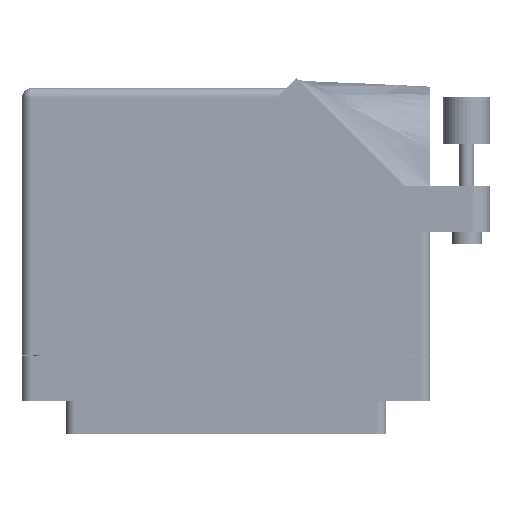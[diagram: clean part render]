
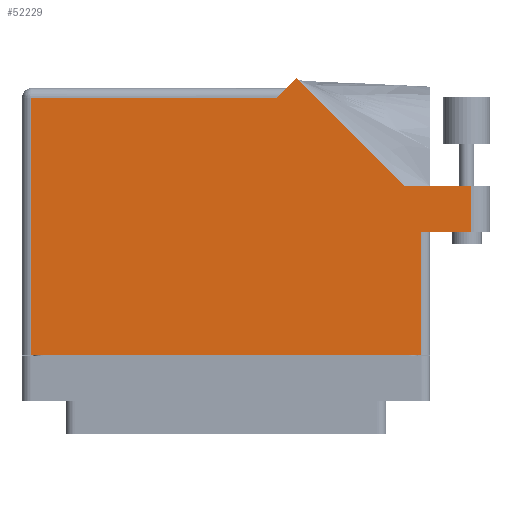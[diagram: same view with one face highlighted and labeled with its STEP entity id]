
A CAD part, front view. The second image highlights one B-rep face of the part: STEP entity #52229.
In plain terms, the highlighted face is planar.
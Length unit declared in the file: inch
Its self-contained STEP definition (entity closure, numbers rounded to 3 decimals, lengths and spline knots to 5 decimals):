
#177 = CARTESIAN_POINT ( 'NONE',  ( 0.46971, 1.74571, 0.617 ) ) ;
#880 = CARTESIAN_POINT ( 'NONE',  ( -1.359, -0.1, 0.617 ) ) ;
#1022 = EDGE_CURVE ( 'NONE', #62810, #7657, #22657, .T. ) ;
#1053 = CARTESIAN_POINT ( 'NONE',  ( -1.297, 1.613, 0.617 ) ) ;
#2074 = CARTESIAN_POINT ( 'NONE',  ( 0.337, 1.613, 0.617 ) ) ;
#2374 = ORIENTED_EDGE ( 'NONE', *, *, #52291, .T. ) ;
#2992 = ORIENTED_EDGE ( 'NONE', *, *, #36825, .T. ) ;
#3361 = LINE ( 'NONE', #880, #59440 ) ;
#3631 = CARTESIAN_POINT ( 'NONE',  ( 1.19342, 1.022, 0.617 ) ) ;
#3835 = LINE ( 'NONE', #46637, #49665 ) ;
#4094 = VERTEX_POINT ( 'NONE', #69458 ) ;
#4654 = EDGE_CURVE ( 'NONE', #60311, #33044, #35469, .T. ) ;
#4778 = ORIENTED_EDGE ( 'NONE', *, *, #31855, .T. ) ;
#5487 = VECTOR ( 'NONE', #17657, 39.37008 ) ;
#6128 = LINE ( 'NONE', #58465, #59645 ) ;
#6171 = CARTESIAN_POINT ( 'NONE',  ( -1.359, 1.675, 0.617 ) ) ;
#6475 = ORIENTED_EDGE ( 'NONE', *, *, #55195, .T. ) ;
#7368 = EDGE_CURVE ( 'NONE', #4094, #60311, #11407, .T. ) ;
#7657 = VERTEX_POINT ( 'NONE', #1053 ) ;
#7923 = AXIS2_PLACEMENT_3D ( 'NONE', #6171, #37727, #27763 ) ;
#8022 = DIRECTION ( 'NONE',  ( -0.707, -0.707, 0. ) ) ;
#10796 = CARTESIAN_POINT ( 'NONE',  ( 1.297, 0.715, 0.617 ) ) ;
#11407 = LINE ( 'NONE', #41815, #5487 ) ;
#14910 = LINE ( 'NONE', #33439, #36952 ) ;
#15592 = ORIENTED_EDGE ( 'NONE', *, *, #4654, .T. ) ;
#17074 = PLANE ( 'NONE',  #7923 ) ;
#17657 = DIRECTION ( 'NONE',  ( -1., 0., 0. ) ) ;
#18263 = CARTESIAN_POINT ( 'NONE',  ( 1.19342, 1.022, 0.617 ) ) ;
#18620 = VECTOR ( 'NONE', #52535, 39.37008 ) ;
#22469 = CARTESIAN_POINT ( 'NONE',  ( 1.359, 0.715, 0.617 ) ) ;
#22657 = LINE ( 'NONE', #40861, #48982 ) ;
#25996 = VERTEX_POINT ( 'NONE', #70314 ) ;
#27763 = DIRECTION ( 'NONE',  ( -1., 0., 0. ) ) ;
#28224 = VECTOR ( 'NONE', #50427, 39.37008 ) ;
#29945 = CARTESIAN_POINT ( 'NONE',  ( 1.297, -0.1, 0.617 ) ) ;
#30753 = VECTOR ( 'NONE', #45112, 39.37008 ) ;
#31855 = EDGE_CURVE ( 'NONE', #43001, #4094, #6128, .T. ) ;
#33044 = VERTEX_POINT ( 'NONE', #177 ) ;
#33072 = ORIENTED_EDGE ( 'NONE', *, *, #66696, .T. ) ;
#33439 = CARTESIAN_POINT ( 'NONE',  ( -1.297, -0.1, 0.617 ) ) ;
#34406 = DIRECTION ( 'NONE',  ( 0., -1., 0. ) ) ;
#35387 = VERTEX_POINT ( 'NONE', #63617 ) ;
#35469 = LINE ( 'NONE', #3631, #18620 ) ;
#36139 = FACE_OUTER_BOUND ( 'NONE', #67970, .T. ) ;
#36825 = EDGE_CURVE ( 'NONE', #25996, #43001, #40130, .T. ) ;
#36952 = VECTOR ( 'NONE', #34406, 39.37008 ) ;
#37727 = DIRECTION ( 'NONE',  ( 0., 0., -1. ) ) ;
#40130 = LINE ( 'NONE', #22469, #28224 ) ;
#40861 = CARTESIAN_POINT ( 'NONE',  ( -1.359, 1.613, 0.617 ) ) ;
#41815 = CARTESIAN_POINT ( 'NONE',  ( 1.759, 1.022, 0.617 ) ) ;
#43001 = VERTEX_POINT ( 'NONE', #66863 ) ;
#45112 = DIRECTION ( 'NONE',  ( 0., 1., 0. ) ) ;
#46322 = ORIENTED_EDGE ( 'NONE', *, *, #1022, .T. ) ;
#46637 = CARTESIAN_POINT ( 'NONE',  ( 0.399, 1.675, 0.617 ) ) ;
#47023 = DIRECTION ( 'NONE',  ( 0., 1., 0. ) ) ;
#48982 = VECTOR ( 'NONE', #62781, 39.37008 ) ;
#49665 = VECTOR ( 'NONE', #8022, 39.37008 ) ;
#50427 = DIRECTION ( 'NONE',  ( 1., 0., 0. ) ) ;
#52229 = ADVANCED_FACE ( 'NONE', ( #36139 ), #17074, .F. ) ;
#52291 = EDGE_CURVE ( 'NONE', #7657, #35387, #14910, .T. ) ;
#52535 = DIRECTION ( 'NONE',  ( -0.707, 0.707, 0. ) ) ;
#55195 = EDGE_CURVE ( 'NONE', #58256, #25996, #59667, .T. ) ;
#55841 = ORIENTED_EDGE ( 'NONE', *, *, #7368, .T. ) ;
#55918 = EDGE_CURVE ( 'NONE', #33044, #62810, #3835, .T. ) ;
#57486 = DIRECTION ( 'NONE',  ( 1., 0., 0. ) ) ;
#58256 = VERTEX_POINT ( 'NONE', #29945 ) ;
#58465 = CARTESIAN_POINT ( 'NONE',  ( 1.634, 1.022, 0.617 ) ) ;
#59440 = VECTOR ( 'NONE', #57486, 39.37008 ) ;
#59645 = VECTOR ( 'NONE', #47023, 39.37008 ) ;
#59667 = LINE ( 'NONE', #10796, #30753 ) ;
#60311 = VERTEX_POINT ( 'NONE', #18263 ) ;
#62781 = DIRECTION ( 'NONE',  ( -1., 0., 0. ) ) ;
#62810 = VERTEX_POINT ( 'NONE', #2074 ) ;
#63617 = CARTESIAN_POINT ( 'NONE',  ( -1.297, -0.1, 0.617 ) ) ;
#66696 = EDGE_CURVE ( 'NONE', #35387, #58256, #3361, .T. ) ;
#66863 = CARTESIAN_POINT ( 'NONE',  ( 1.634, 0.715, 0.617 ) ) ;
#67970 = EDGE_LOOP ( 'NONE', ( #2992, #4778, #55841, #15592, #70456, #46322, #2374, #33072, #6475 ) ) ;
#69458 = CARTESIAN_POINT ( 'NONE',  ( 1.634, 1.022, 0.617 ) ) ;
#70314 = CARTESIAN_POINT ( 'NONE',  ( 1.297, 0.715, 0.617 ) ) ;
#70456 = ORIENTED_EDGE ( 'NONE', *, *, #55918, .T. ) ;
